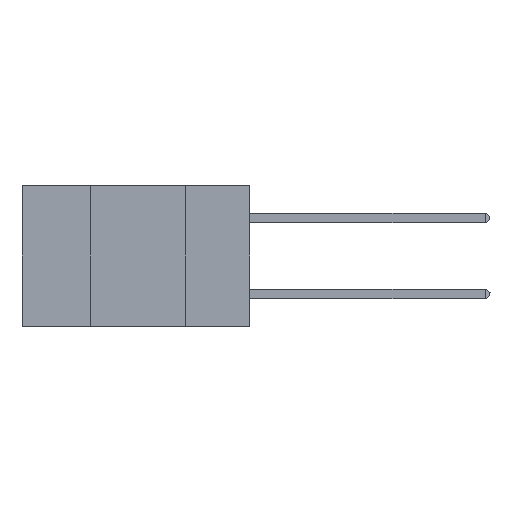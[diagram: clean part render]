
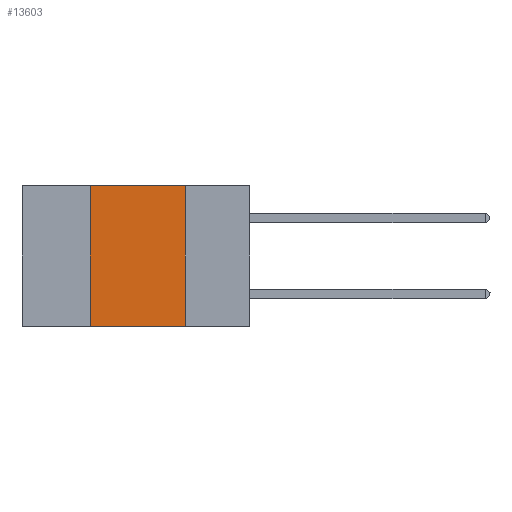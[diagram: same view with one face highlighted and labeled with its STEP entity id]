
A CAD part, left-side view. The second image highlights one B-rep face of the part: STEP entity #13603.
In plain terms, the highlighted planar face has unit normal (-1, 0, 0).
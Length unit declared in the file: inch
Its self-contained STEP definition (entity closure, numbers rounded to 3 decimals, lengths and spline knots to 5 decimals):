
#113 = VECTOR ( 'NONE', #516, 39.37008 ) ;
#218 = ORIENTED_EDGE ( 'NONE', *, *, #13431, .F. ) ;
#516 = DIRECTION ( 'NONE',  ( 0., 0., 1. ) ) ;
#801 = AXIS2_PLACEMENT_3D ( 'NONE', #2690, #12176, #10429 ) ;
#969 = DIRECTION ( 'NONE',  ( 0., -1., 0. ) ) ;
#2018 = EDGE_CURVE ( 'NONE', #14673, #18165, #7955, .T. ) ;
#2690 = CARTESIAN_POINT ( 'NONE',  ( 0., 0.6, 0. ) ) ;
#3661 = VERTEX_POINT ( 'NONE', #12726 ) ;
#4445 = VECTOR ( 'NONE', #5424, 39.37008 ) ;
#5284 = ORIENTED_EDGE ( 'NONE', *, *, #12953, .F. ) ;
#5424 = DIRECTION ( 'NONE',  ( 0., -1., 0. ) ) ;
#5608 = FACE_OUTER_BOUND ( 'NONE', #15824, .T. ) ;
#6053 = ORIENTED_EDGE ( 'NONE', *, *, #2018, .F. ) ;
#7810 = VECTOR ( 'NONE', #969, 39.37008 ) ;
#7819 = EDGE_CURVE ( 'NONE', #19009, #18165, #10270, .T. ) ;
#7930 = ORIENTED_EDGE ( 'NONE', *, *, #7819, .T. ) ;
#7955 = LINE ( 'NONE', #17301, #9675 ) ;
#8319 = CARTESIAN_POINT ( 'NONE',  ( 0., 0.42, 0. ) ) ;
#9675 = VECTOR ( 'NONE', #14292, 39.37008 ) ;
#10270 = LINE ( 'NONE', #13261, #7810 ) ;
#10429 = DIRECTION ( 'NONE',  ( 0., 0., -1. ) ) ;
#11288 = LINE ( 'NONE', #17585, #4445 ) ;
#12176 = DIRECTION ( 'NONE',  ( 1., 0., 0. ) ) ;
#12726 = CARTESIAN_POINT ( 'NONE',  ( 0., 0.42, 0. ) ) ;
#12814 = CARTESIAN_POINT ( 'NONE',  ( 0., 0.17, 0. ) ) ;
#12953 = EDGE_CURVE ( 'NONE', #3661, #14673, #11288, .T. ) ;
#13261 = CARTESIAN_POINT ( 'NONE',  ( 0., 0.6, -0.37 ) ) ;
#13314 = LINE ( 'NONE', #8319, #113 ) ;
#13431 = EDGE_CURVE ( 'NONE', #19009, #3661, #13314, .T. ) ;
#13603 = ADVANCED_FACE ( 'NONE', ( #5608 ), #20166, .F. ) ;
#14292 = DIRECTION ( 'NONE',  ( 0., 0., -1. ) ) ;
#14673 = VERTEX_POINT ( 'NONE', #12814 ) ;
#15824 = EDGE_LOOP ( 'NONE', ( #6053, #5284, #218, #7930 ) ) ;
#17301 = CARTESIAN_POINT ( 'NONE',  ( 0., 0.17, 0. ) ) ;
#17585 = CARTESIAN_POINT ( 'NONE',  ( 0., 0.6, 0. ) ) ;
#18165 = VERTEX_POINT ( 'NONE', #18311 ) ;
#18311 = CARTESIAN_POINT ( 'NONE',  ( 0., 0.17, -0.37 ) ) ;
#19009 = VERTEX_POINT ( 'NONE', #19305 ) ;
#19305 = CARTESIAN_POINT ( 'NONE',  ( 0., 0.42, -0.37 ) ) ;
#20166 = PLANE ( 'NONE',  #801 ) ;
